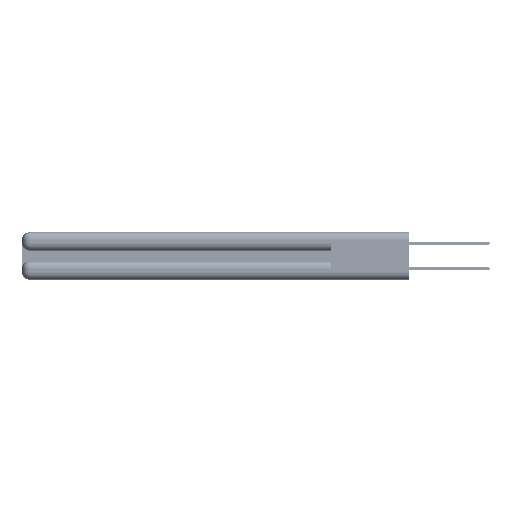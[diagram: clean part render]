
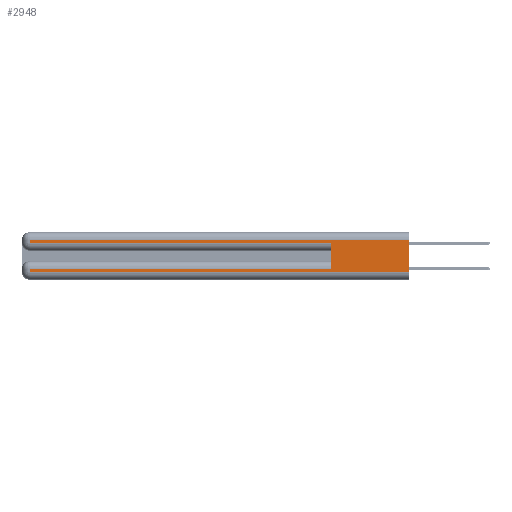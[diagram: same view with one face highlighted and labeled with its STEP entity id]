
A CAD part, left-side view. The second image highlights one B-rep face of the part: STEP entity #2948.
In plain terms, the highlighted planar face has unit normal (-1, 0, 0).
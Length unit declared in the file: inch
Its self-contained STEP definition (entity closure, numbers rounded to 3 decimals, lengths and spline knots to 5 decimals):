
#539 = DIRECTION ( 'NONE',  ( 0., 0., -1. ) ) ;
#1122 = DIRECTION ( 'NONE',  ( 0., 1., 0. ) ) ;
#2492 = VERTEX_POINT ( 'NONE', #30124 ) ;
#2948 = ADVANCED_FACE ( 'NONE', ( #7446 ), #33115, .F. ) ;
#3318 = EDGE_CURVE ( 'NONE', #2492, #50933, #28257, .T. ) ;
#4517 = VECTOR ( 'NONE', #15011, 39.37008 ) ;
#6800 = VECTOR ( 'NONE', #31542, 39.37008 ) ;
#7344 = DIRECTION ( 'NONE',  ( 1., 0., 0. ) ) ;
#7446 = FACE_OUTER_BOUND ( 'NONE', #23496, .T. ) ;
#7591 = EDGE_CURVE ( 'NONE', #19159, #17842, #20024, .T. ) ;
#7679 = ORIENTED_EDGE ( 'NONE', *, *, #18879, .F. ) ;
#8005 = CARTESIAN_POINT ( 'NONE',  ( 0., 2.94, 0.31 ) ) ;
#9173 = DIRECTION ( 'NONE',  ( 0., -1., 0. ) ) ;
#10092 = VECTOR ( 'NONE', #37022, 39.37008 ) ;
#10145 = VERTEX_POINT ( 'NONE', #46100 ) ;
#11259 = CARTESIAN_POINT ( 'NONE',  ( 0., 2.94, 0.37 ) ) ;
#11677 = DIRECTION ( 'NONE',  ( 0., 0., -1. ) ) ;
#13948 = ORIENTED_EDGE ( 'NONE', *, *, #41630, .T. ) ;
#15011 = DIRECTION ( 'NONE',  ( 0., 0., -1. ) ) ;
#16397 = LINE ( 'NONE', #17467, #24461 ) ;
#17467 = CARTESIAN_POINT ( 'NONE',  ( 0., 0., 0.285 ) ) ;
#17842 = VERTEX_POINT ( 'NONE', #21292 ) ;
#18704 = VECTOR ( 'NONE', #1122, 39.37008 ) ;
#18879 = EDGE_CURVE ( 'NONE', #34493, #10145, #45258, .T. ) ;
#19159 = VERTEX_POINT ( 'NONE', #8005 ) ;
#19333 = EDGE_CURVE ( 'NONE', #36150, #19159, #49890, .T. ) ;
#19338 = CARTESIAN_POINT ( 'NONE',  ( 0., 2.94, 0.37 ) ) ;
#20024 = LINE ( 'NONE', #19338, #4517 ) ;
#21268 = LINE ( 'NONE', #43304, #31364 ) ;
#21292 = CARTESIAN_POINT ( 'NONE',  ( 0., 2.94, 0.285 ) ) ;
#22173 = VERTEX_POINT ( 'NONE', #49197 ) ;
#22768 = LINE ( 'NONE', #32196, #42298 ) ;
#23406 = ORIENTED_EDGE ( 'NONE', *, *, #19333, .T. ) ;
#23496 = EDGE_LOOP ( 'NONE', ( #36018, #23406, #24131, #13948, #7679, #45262, #27483, #54355 ) ) ;
#24131 = ORIENTED_EDGE ( 'NONE', *, *, #7591, .T. ) ;
#24301 = CARTESIAN_POINT ( 'NONE',  ( 0., 2.94, 0.06 ) ) ;
#24430 = CARTESIAN_POINT ( 'NONE',  ( 0., 0., 0.31 ) ) ;
#24461 = VECTOR ( 'NONE', #9173, 39.37008 ) ;
#24762 = EDGE_CURVE ( 'NONE', #50933, #22173, #22768, .T. ) ;
#26721 = CARTESIAN_POINT ( 'NONE',  ( 0., 0., 0.085 ) ) ;
#27118 = DIRECTION ( 'NONE',  ( 0., -1., 0. ) ) ;
#27444 = AXIS2_PLACEMENT_3D ( 'NONE', #32920, #7344, #11677 ) ;
#27483 = ORIENTED_EDGE ( 'NONE', *, *, #3318, .T. ) ;
#28257 = LINE ( 'NONE', #11259, #10092 ) ;
#30124 = CARTESIAN_POINT ( 'NONE',  ( 0., 2.94, 0.085 ) ) ;
#31364 = VECTOR ( 'NONE', #539, 39.37008 ) ;
#31542 = DIRECTION ( 'NONE',  ( 0., 1., 0. ) ) ;
#32196 = CARTESIAN_POINT ( 'NONE',  ( 0., 0., 0.06 ) ) ;
#32442 = VECTOR ( 'NONE', #44922, 39.37008 ) ;
#32920 = CARTESIAN_POINT ( 'NONE',  ( 0., 0., 0.37 ) ) ;
#33115 = PLANE ( 'NONE',  #27444 ) ;
#33457 = LINE ( 'NONE', #26721, #18704 ) ;
#34237 = EDGE_CURVE ( 'NONE', #36150, #22173, #21268, .T. ) ;
#34493 = VERTEX_POINT ( 'NONE', #54317 ) ;
#36018 = ORIENTED_EDGE ( 'NONE', *, *, #34237, .F. ) ;
#36058 = CARTESIAN_POINT ( 'NONE',  ( 0., 0.6, 0.145 ) ) ;
#36150 = VERTEX_POINT ( 'NONE', #24430 ) ;
#37022 = DIRECTION ( 'NONE',  ( 0., 0., -1. ) ) ;
#41630 = EDGE_CURVE ( 'NONE', #17842, #10145, #16397, .T. ) ;
#42298 = VECTOR ( 'NONE', #27118, 39.37008 ) ;
#43304 = CARTESIAN_POINT ( 'NONE',  ( 0., 0., 0.37 ) ) ;
#44922 = DIRECTION ( 'NONE',  ( 0., 0., 1. ) ) ;
#45258 = LINE ( 'NONE', #36058, #32442 ) ;
#45262 = ORIENTED_EDGE ( 'NONE', *, *, #47876, .T. ) ;
#46100 = CARTESIAN_POINT ( 'NONE',  ( 0., 0.6, 0.285 ) ) ;
#47876 = EDGE_CURVE ( 'NONE', #34493, #2492, #33457, .T. ) ;
#49197 = CARTESIAN_POINT ( 'NONE',  ( 0., 0., 0.06 ) ) ;
#49890 = LINE ( 'NONE', #51144, #6800 ) ;
#50933 = VERTEX_POINT ( 'NONE', #24301 ) ;
#51144 = CARTESIAN_POINT ( 'NONE',  ( 0., 0., 0.31 ) ) ;
#54317 = CARTESIAN_POINT ( 'NONE',  ( 0., 0.6, 0.085 ) ) ;
#54355 = ORIENTED_EDGE ( 'NONE', *, *, #24762, .T. ) ;
